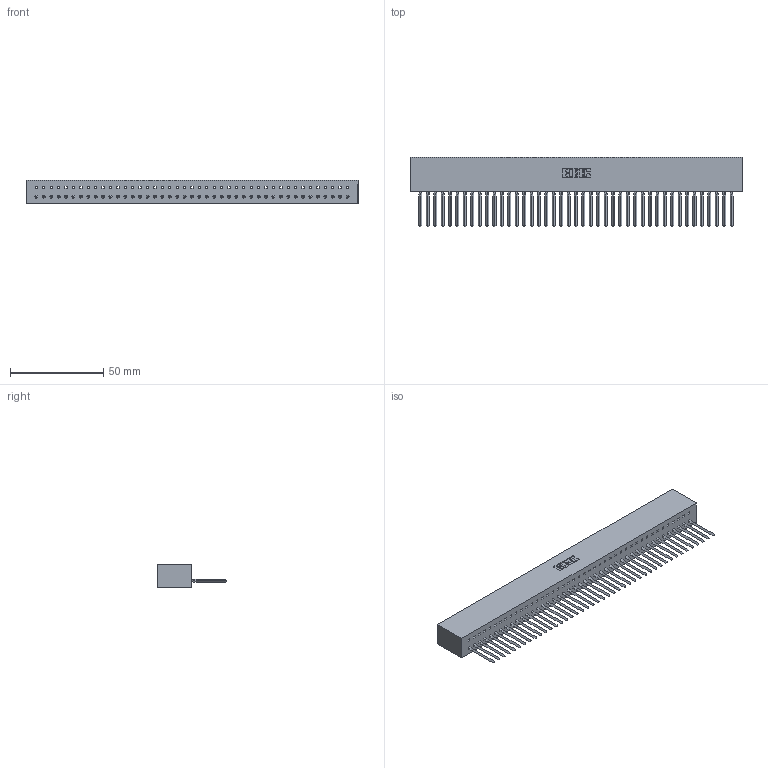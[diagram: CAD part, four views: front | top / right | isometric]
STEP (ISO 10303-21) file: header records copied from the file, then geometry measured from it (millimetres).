
FILE_DESCRIPTION (( 'STEP AP203' ), '1' );
FILE_NAME ('317-043-542-601.STEP', '2020-02-28T01:39:45', ( '' ), ( '' ), 'SwSTEP 2.0', 'SolidWorks 2016', '' );
FILE_SCHEMA (( 'CONFIG_CONTROL_DESIGN' ));
Length unit declared in the file: inch
Products named in the file (3): 317-290-003_542; 317-043-542-601; 317 Part_Lugless
Assembly tree (44 placements, depth 2):
  317-043-542-601
    317 Part_Lugless
    317-290-003_542  x43
Bounding box: 177.6 x 37.34 x 12.7 mm (x, y, z)
Volume: 29047.1 mm3; surface area: 35497.4 mm2
Topology: 44 solids, 44 shells, 3315 faces, 9570 edges, 6178 vertices
Faces by surface type: plane 2802, cylinder 341, bspline 172
Entity records: 59249 total; most frequent: CARTESIAN_POINT 10782, ORIENTED_EDGE 10488, DIRECTION 8726, EDGE_CURVE 5244, VECTOR 5082, LINE 5082, VERTEX_POINT 3490, AXIS2_PLACEMENT_3D 1822
